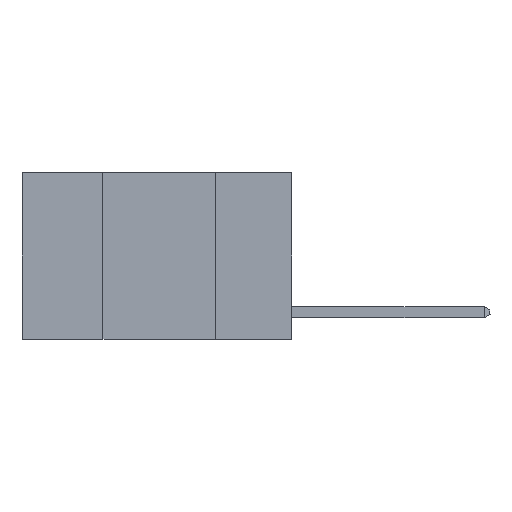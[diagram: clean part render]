
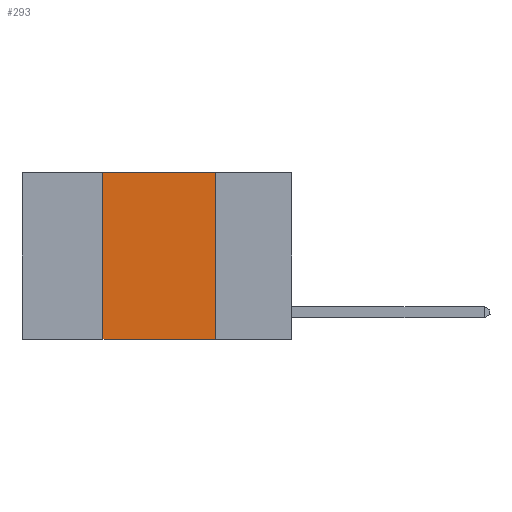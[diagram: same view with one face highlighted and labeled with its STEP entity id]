
A CAD part, left-side view. The second image highlights one B-rep face of the part: STEP entity #293.
In plain terms, the highlighted planar face has unit normal (-1, 0, 0).
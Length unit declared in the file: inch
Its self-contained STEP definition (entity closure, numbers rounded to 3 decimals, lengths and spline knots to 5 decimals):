
#110 = EDGE_CURVE ( 'NONE', #1927, #9441, #3525, .T. ) ;
#293 = ADVANCED_FACE ( 'NONE', ( #3401 ), #7667, .F. ) ;
#818 = CARTESIAN_POINT ( 'NONE',  ( 0., 0.6, 0. ) ) ;
#1106 = CARTESIAN_POINT ( 'NONE',  ( 0., 0.17, -0.37 ) ) ;
#1320 = ORIENTED_EDGE ( 'NONE', *, *, #6916, .F. ) ;
#1401 = VECTOR ( 'NONE', #8181, 39.37008 ) ;
#1627 = DIRECTION ( 'NONE',  ( 0., -1., 0. ) ) ;
#1784 = LINE ( 'NONE', #7548, #1401 ) ;
#1927 = VERTEX_POINT ( 'NONE', #6891 ) ;
#2200 = DIRECTION ( 'NONE',  ( 0., -1., 0. ) ) ;
#2950 = CARTESIAN_POINT ( 'NONE',  ( 0., 0.6, -0.37 ) ) ;
#3401 = FACE_OUTER_BOUND ( 'NONE', #7855, .T. ) ;
#3525 = LINE ( 'NONE', #2950, #7190 ) ;
#3650 = LINE ( 'NONE', #818, #5165 ) ;
#4021 = DIRECTION ( 'NONE',  ( 1., 0., 0. ) ) ;
#4317 = CARTESIAN_POINT ( 'NONE',  ( 0., 0.17, 0. ) ) ;
#4798 = DIRECTION ( 'NONE',  ( 0., 0., -1. ) ) ;
#5090 = EDGE_CURVE ( 'NONE', #7264, #9441, #1784, .T. ) ;
#5165 = VECTOR ( 'NONE', #1627, 39.37008 ) ;
#5172 = CARTESIAN_POINT ( 'NONE',  ( 0., 0.42, 0. ) ) ;
#6605 = ORIENTED_EDGE ( 'NONE', *, *, #5090, .F. ) ;
#6699 = VERTEX_POINT ( 'NONE', #7284 ) ;
#6879 = EDGE_CURVE ( 'NONE', #6699, #7264, #3650, .T. ) ;
#6891 = CARTESIAN_POINT ( 'NONE',  ( 0., 0.42, -0.37 ) ) ;
#6916 = EDGE_CURVE ( 'NONE', #1927, #6699, #7959, .T. ) ;
#7043 = ORIENTED_EDGE ( 'NONE', *, *, #110, .T. ) ;
#7190 = VECTOR ( 'NONE', #2200, 39.37008 ) ;
#7264 = VERTEX_POINT ( 'NONE', #4317 ) ;
#7284 = CARTESIAN_POINT ( 'NONE',  ( 0., 0.42, 0. ) ) ;
#7298 = AXIS2_PLACEMENT_3D ( 'NONE', #8302, #4021, #4798 ) ;
#7322 = ORIENTED_EDGE ( 'NONE', *, *, #6879, .F. ) ;
#7350 = DIRECTION ( 'NONE',  ( 0., 0., 1. ) ) ;
#7548 = CARTESIAN_POINT ( 'NONE',  ( 0., 0.17, 0. ) ) ;
#7667 = PLANE ( 'NONE',  #7298 ) ;
#7737 = VECTOR ( 'NONE', #7350, 39.37008 ) ;
#7855 = EDGE_LOOP ( 'NONE', ( #6605, #7322, #1320, #7043 ) ) ;
#7959 = LINE ( 'NONE', #5172, #7737 ) ;
#8181 = DIRECTION ( 'NONE',  ( 0., 0., -1. ) ) ;
#8302 = CARTESIAN_POINT ( 'NONE',  ( 0., 0.6, 0. ) ) ;
#9441 = VERTEX_POINT ( 'NONE', #1106 ) ;
